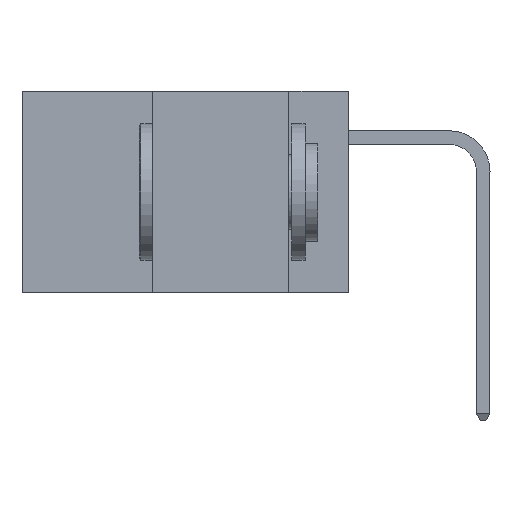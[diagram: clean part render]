
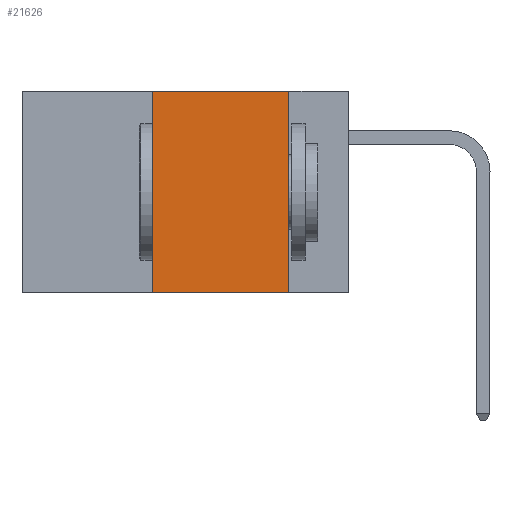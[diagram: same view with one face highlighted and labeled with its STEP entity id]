
A CAD part, left-side view. The second image highlights one B-rep face of the part: STEP entity #21626.
In plain terms, the highlighted planar face has unit normal (-1, 0, 0).
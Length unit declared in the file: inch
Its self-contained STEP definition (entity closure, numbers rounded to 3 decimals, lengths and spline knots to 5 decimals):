
#1344 = ORIENTED_EDGE ( 'NONE', *, *, #16906, .F. ) ;
#1785 = LINE ( 'NONE', #27345, #9763 ) ;
#2870 = VERTEX_POINT ( 'NONE', #35717 ) ;
#2909 = DIRECTION ( 'NONE',  ( 0., -1., 0. ) ) ;
#3474 = DIRECTION ( 'NONE',  ( 0., -1., 0. ) ) ;
#4956 = LINE ( 'NONE', #38614, #11928 ) ;
#5363 = VERTEX_POINT ( 'NONE', #30198 ) ;
#7193 = EDGE_CURVE ( 'NONE', #17561, #2870, #1785, .T. ) ;
#7319 = ORIENTED_EDGE ( 'NONE', *, *, #24215, .F. ) ;
#9763 = VECTOR ( 'NONE', #3474, 39.37008 ) ;
#9850 = DIRECTION ( 'NONE',  ( 0., 0., -1. ) ) ;
#10828 = CARTESIAN_POINT ( 'NONE',  ( 0., 0.36, -0.37 ) ) ;
#11714 = EDGE_LOOP ( 'NONE', ( #7319, #24296, #1344, #13431 ) ) ;
#11928 = VECTOR ( 'NONE', #2909, 39.37008 ) ;
#12485 = DIRECTION ( 'NONE',  ( 1., 0., 0. ) ) ;
#13431 = ORIENTED_EDGE ( 'NONE', *, *, #7193, .T. ) ;
#16906 = EDGE_CURVE ( 'NONE', #17561, #20838, #36245, .T. ) ;
#17561 = VERTEX_POINT ( 'NONE', #10828 ) ;
#17821 = VECTOR ( 'NONE', #9850, 39.37008 ) ;
#19394 = FACE_OUTER_BOUND ( 'NONE', #11714, .T. ) ;
#20838 = VERTEX_POINT ( 'NONE', #32774 ) ;
#21626 = ADVANCED_FACE ( 'NONE', ( #19394 ), #30362, .F. ) ;
#21725 = CARTESIAN_POINT ( 'NONE',  ( 0., 0.11, 0. ) ) ;
#22335 = DIRECTION ( 'NONE',  ( 0., 0., 1. ) ) ;
#23912 = AXIS2_PLACEMENT_3D ( 'NONE', #24382, #12485, #33350 ) ;
#24215 = EDGE_CURVE ( 'NONE', #5363, #2870, #25756, .T. ) ;
#24296 = ORIENTED_EDGE ( 'NONE', *, *, #35713, .F. ) ;
#24382 = CARTESIAN_POINT ( 'NONE',  ( 0., 0.6, 0. ) ) ;
#25756 = LINE ( 'NONE', #21725, #17821 ) ;
#27345 = CARTESIAN_POINT ( 'NONE',  ( 0., 0.6, -0.37 ) ) ;
#28221 = CARTESIAN_POINT ( 'NONE',  ( 0., 0.36, 0. ) ) ;
#30198 = CARTESIAN_POINT ( 'NONE',  ( 0., 0.11, 0. ) ) ;
#30362 = PLANE ( 'NONE',  #23912 ) ;
#32774 = CARTESIAN_POINT ( 'NONE',  ( 0., 0.36, 0. ) ) ;
#33350 = DIRECTION ( 'NONE',  ( 0., 0., -1. ) ) ;
#35315 = VECTOR ( 'NONE', #22335, 39.37008 ) ;
#35713 = EDGE_CURVE ( 'NONE', #20838, #5363, #4956, .T. ) ;
#35717 = CARTESIAN_POINT ( 'NONE',  ( 0., 0.11, -0.37 ) ) ;
#36245 = LINE ( 'NONE', #28221, #35315 ) ;
#38614 = CARTESIAN_POINT ( 'NONE',  ( 0., 0.6, 0. ) ) ;
